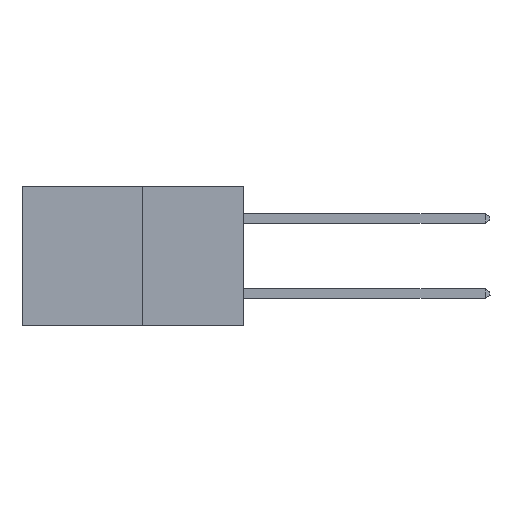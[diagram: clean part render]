
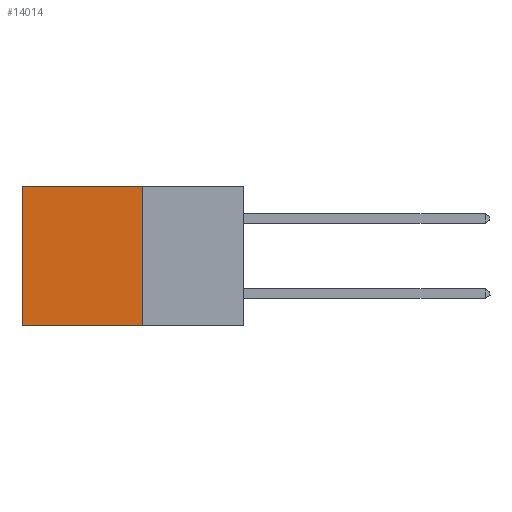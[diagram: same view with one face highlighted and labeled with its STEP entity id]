
A CAD part, left-side view. The second image highlights one B-rep face of the part: STEP entity #14014.
In plain terms, the highlighted planar face has unit normal (-1, 0, 0).
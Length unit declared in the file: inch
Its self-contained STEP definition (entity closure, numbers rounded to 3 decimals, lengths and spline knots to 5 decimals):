
#2109 = VERTEX_POINT ( 'NONE', #16372 ) ;
#2918 = EDGE_CURVE ( 'NONE', #2109, #15733, #14529, .T. ) ;
#3153 = DIRECTION ( 'NONE',  ( 0., 0., -1. ) ) ;
#3304 = DIRECTION ( 'NONE',  ( 1., 0., 0. ) ) ;
#3635 = CARTESIAN_POINT ( 'NONE',  ( 0.277, 0.27, 0. ) ) ;
#5825 = CARTESIAN_POINT ( 'NONE',  ( 0.277, 0.59, -0.37 ) ) ;
#6465 = ORIENTED_EDGE ( 'NONE', *, *, #12130, .T. ) ;
#8125 = ORIENTED_EDGE ( 'NONE', *, *, #20743, .F. ) ;
#8755 = CARTESIAN_POINT ( 'NONE',  ( 0.277, 0.27, -0.37 ) ) ;
#8783 = ORIENTED_EDGE ( 'NONE', *, *, #2918, .T. ) ;
#11747 = CARTESIAN_POINT ( 'NONE',  ( 0.277, 0.59, -0.37 ) ) ;
#12130 = EDGE_CURVE ( 'NONE', #15009, #2109, #24703, .T. ) ;
#12472 = VECTOR ( 'NONE', #15838, 39.37008 ) ;
#13284 = DIRECTION ( 'NONE',  ( 0., 1., 0. ) ) ;
#13929 = VECTOR ( 'NONE', #3153, 39.37008 ) ;
#14014 = ADVANCED_FACE ( 'NONE', ( #23424 ), #22570, .F. ) ;
#14529 = LINE ( 'NONE', #5825, #13929 ) ;
#15009 = VERTEX_POINT ( 'NONE', #15671 ) ;
#15300 = AXIS2_PLACEMENT_3D ( 'NONE', #24480, #3304, #16864 ) ;
#15318 = VERTEX_POINT ( 'NONE', #8755 ) ;
#15671 = CARTESIAN_POINT ( 'NONE',  ( 0.277, 0.27, 0. ) ) ;
#15733 = VERTEX_POINT ( 'NONE', #11747 ) ;
#15838 = DIRECTION ( 'NONE',  ( 0., 0., -1. ) ) ;
#15882 = CARTESIAN_POINT ( 'NONE',  ( 0.277, 0.27, -0.37 ) ) ;
#16372 = CARTESIAN_POINT ( 'NONE',  ( 0.277, 0.59, 0. ) ) ;
#16864 = DIRECTION ( 'NONE',  ( 0., 0., -1. ) ) ;
#17637 = LINE ( 'NONE', #23494, #12472 ) ;
#17842 = DIRECTION ( 'NONE',  ( 0., 1., 0. ) ) ;
#19041 = VECTOR ( 'NONE', #13284, 39.37008 ) ;
#19745 = ORIENTED_EDGE ( 'NONE', *, *, #24887, .F. ) ;
#20743 = EDGE_CURVE ( 'NONE', #15318, #15733, #23640, .T. ) ;
#22447 = VECTOR ( 'NONE', #17842, 39.37008 ) ;
#22570 = PLANE ( 'NONE',  #15300 ) ;
#23151 = EDGE_LOOP ( 'NONE', ( #8783, #8125, #19745, #6465 ) ) ;
#23424 = FACE_OUTER_BOUND ( 'NONE', #23151, .T. ) ;
#23494 = CARTESIAN_POINT ( 'NONE',  ( 0.277, 0.27, -0.37 ) ) ;
#23640 = LINE ( 'NONE', #15882, #22447 ) ;
#24480 = CARTESIAN_POINT ( 'NONE',  ( 0.277, 0.27, -0.37 ) ) ;
#24703 = LINE ( 'NONE', #3635, #19041 ) ;
#24887 = EDGE_CURVE ( 'NONE', #15009, #15318, #17637, .T. ) ;
